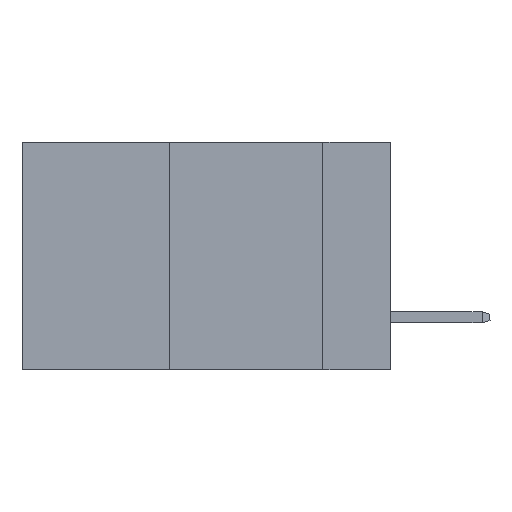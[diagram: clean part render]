
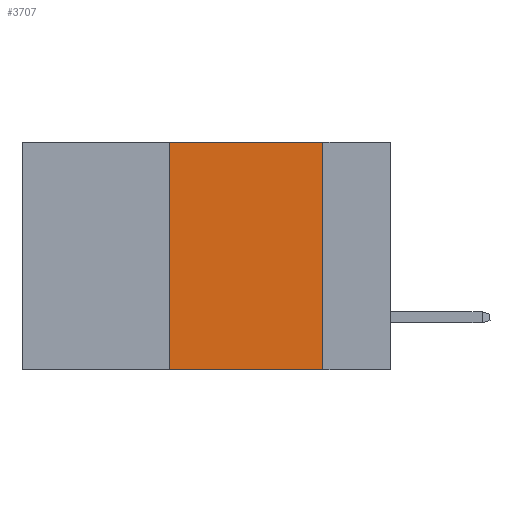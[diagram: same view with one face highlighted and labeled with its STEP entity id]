
A CAD part, left-side view. The second image highlights one B-rep face of the part: STEP entity #3707.
In plain terms, the highlighted planar face has unit normal (-1, 0, 0).
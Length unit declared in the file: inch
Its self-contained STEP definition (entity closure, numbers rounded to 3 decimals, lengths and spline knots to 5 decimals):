
#86 = DIRECTION ( 'NONE',  ( 1., 0., 0. ) ) ;
#320 = CARTESIAN_POINT ( 'NONE',  ( 0., 0.36, -0.37 ) ) ;
#612 = ORIENTED_EDGE ( 'NONE', *, *, #983, .F. ) ;
#798 = AXIS2_PLACEMENT_3D ( 'NONE', #2475, #86, #5585 ) ;
#847 = DIRECTION ( 'NONE',  ( 0., -1., 0. ) ) ;
#983 = EDGE_CURVE ( 'NONE', #10025, #1002, #8734, .T. ) ;
#1002 = VERTEX_POINT ( 'NONE', #3250 ) ;
#1820 = VERTEX_POINT ( 'NONE', #4469 ) ;
#1870 = ORIENTED_EDGE ( 'NONE', *, *, #6759, .F. ) ;
#2184 = CARTESIAN_POINT ( 'NONE',  ( 0., 0.6, 0. ) ) ;
#2475 = CARTESIAN_POINT ( 'NONE',  ( 0., 0.6, 0. ) ) ;
#2513 = LINE ( 'NONE', #8664, #4570 ) ;
#2574 = FACE_OUTER_BOUND ( 'NONE', #5751, .T. ) ;
#2656 = VERTEX_POINT ( 'NONE', #320 ) ;
#2694 = CARTESIAN_POINT ( 'NONE',  ( 0., 0.6, -0.37 ) ) ;
#3250 = CARTESIAN_POINT ( 'NONE',  ( 0., 0.11, -0.37 ) ) ;
#3271 = DIRECTION ( 'NONE',  ( 0., 0., 1. ) ) ;
#3707 = ADVANCED_FACE ( 'NONE', ( #2574 ), #4810, .F. ) ;
#3994 = CARTESIAN_POINT ( 'NONE',  ( 0., 0.11, 0. ) ) ;
#4073 = DIRECTION ( 'NONE',  ( 0., 0., -1. ) ) ;
#4215 = DIRECTION ( 'NONE',  ( 0., -1., 0. ) ) ;
#4469 = CARTESIAN_POINT ( 'NONE',  ( 0., 0.36, 0. ) ) ;
#4539 = LINE ( 'NONE', #2694, #6363 ) ;
#4570 = VECTOR ( 'NONE', #3271, 39.37008 ) ;
#4810 = PLANE ( 'NONE',  #798 ) ;
#4863 = EDGE_CURVE ( 'NONE', #1820, #10025, #8357, .T. ) ;
#5585 = DIRECTION ( 'NONE',  ( 0., 0., -1. ) ) ;
#5751 = EDGE_LOOP ( 'NONE', ( #612, #9389, #1870, #9265 ) ) ;
#5788 = CARTESIAN_POINT ( 'NONE',  ( 0., 0.11, 0. ) ) ;
#6363 = VECTOR ( 'NONE', #4215, 39.37008 ) ;
#6759 = EDGE_CURVE ( 'NONE', #2656, #1820, #2513, .T. ) ;
#8108 = EDGE_CURVE ( 'NONE', #2656, #1002, #4539, .T. ) ;
#8112 = VECTOR ( 'NONE', #847, 39.37008 ) ;
#8357 = LINE ( 'NONE', #2184, #8112 ) ;
#8496 = VECTOR ( 'NONE', #4073, 39.37008 ) ;
#8664 = CARTESIAN_POINT ( 'NONE',  ( 0., 0.36, 0. ) ) ;
#8734 = LINE ( 'NONE', #5788, #8496 ) ;
#9265 = ORIENTED_EDGE ( 'NONE', *, *, #8108, .T. ) ;
#9389 = ORIENTED_EDGE ( 'NONE', *, *, #4863, .F. ) ;
#10025 = VERTEX_POINT ( 'NONE', #3994 ) ;
